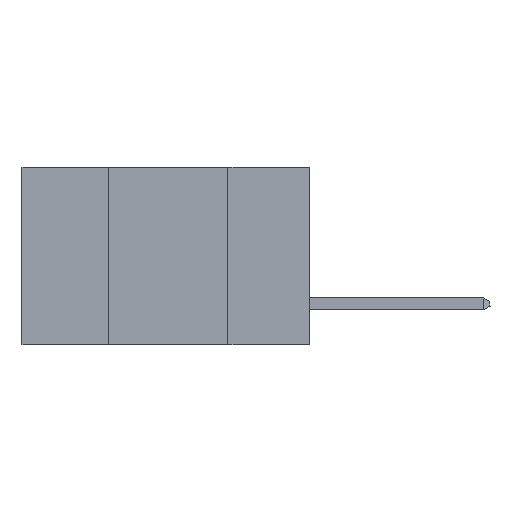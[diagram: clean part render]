
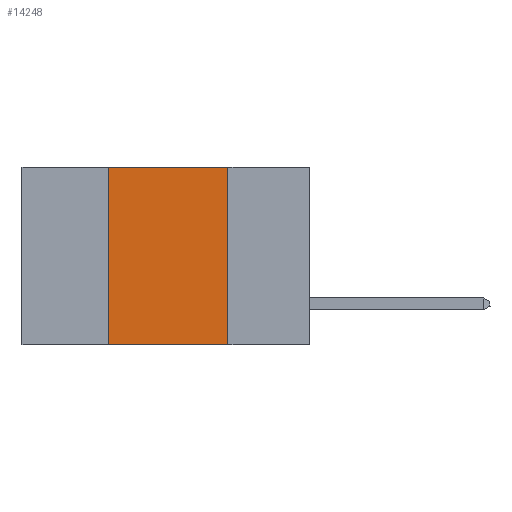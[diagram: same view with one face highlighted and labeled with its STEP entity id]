
A CAD part, left-side view. The second image highlights one B-rep face of the part: STEP entity #14248.
In plain terms, the highlighted planar face has unit normal (-1, 0, 0).
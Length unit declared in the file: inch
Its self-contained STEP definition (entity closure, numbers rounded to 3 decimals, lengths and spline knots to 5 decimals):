
#687 = AXIS2_PLACEMENT_3D ( 'NONE', #15454, #2867, #1609 ) ;
#1334 = EDGE_CURVE ( 'NONE', #13517, #1570, #4063, .T. ) ;
#1570 = VERTEX_POINT ( 'NONE', #13512 ) ;
#1609 = DIRECTION ( 'NONE',  ( 0., 0., -1. ) ) ;
#2159 = LINE ( 'NONE', #13536, #5321 ) ;
#2220 = CARTESIAN_POINT ( 'NONE',  ( 0., 0.42, -0.37 ) ) ;
#2588 = DIRECTION ( 'NONE',  ( 0., -1., 0. ) ) ;
#2867 = DIRECTION ( 'NONE',  ( 1., 0., 0. ) ) ;
#2921 = PLANE ( 'NONE',  #687 ) ;
#3475 = ORIENTED_EDGE ( 'NONE', *, *, #1334, .F. ) ;
#3502 = LINE ( 'NONE', #4851, #13552 ) ;
#4063 = LINE ( 'NONE', #8193, #14668 ) ;
#4851 = CARTESIAN_POINT ( 'NONE',  ( 0., 0.17, 0. ) ) ;
#5321 = VECTOR ( 'NONE', #14844, 39.37008 ) ;
#6093 = DIRECTION ( 'NONE',  ( 0., 0., -1. ) ) ;
#6824 = VERTEX_POINT ( 'NONE', #15093 ) ;
#7123 = CARTESIAN_POINT ( 'NONE',  ( 0., 0.17, 0. ) ) ;
#8193 = CARTESIAN_POINT ( 'NONE',  ( 0., 0.42, 0. ) ) ;
#8251 = DIRECTION ( 'NONE',  ( 0., 0., 1. ) ) ;
#8395 = VECTOR ( 'NONE', #2588, 39.37008 ) ;
#8502 = FACE_OUTER_BOUND ( 'NONE', #9067, .T. ) ;
#9067 = EDGE_LOOP ( 'NONE', ( #9069, #12252, #3475, #12492 ) ) ;
#9069 = ORIENTED_EDGE ( 'NONE', *, *, #9798, .F. ) ;
#9436 = EDGE_CURVE ( 'NONE', #1570, #12215, #2159, .T. ) ;
#9798 = EDGE_CURVE ( 'NONE', #12215, #6824, #3502, .T. ) ;
#11364 = EDGE_CURVE ( 'NONE', #13517, #6824, #15077, .T. ) ;
#12215 = VERTEX_POINT ( 'NONE', #7123 ) ;
#12252 = ORIENTED_EDGE ( 'NONE', *, *, #9436, .F. ) ;
#12492 = ORIENTED_EDGE ( 'NONE', *, *, #11364, .T. ) ;
#13512 = CARTESIAN_POINT ( 'NONE',  ( 0., 0.42, 0. ) ) ;
#13517 = VERTEX_POINT ( 'NONE', #2220 ) ;
#13536 = CARTESIAN_POINT ( 'NONE',  ( 0., 0.6, 0. ) ) ;
#13552 = VECTOR ( 'NONE', #6093, 39.37008 ) ;
#13936 = CARTESIAN_POINT ( 'NONE',  ( 0., 0.6, -0.37 ) ) ;
#14248 = ADVANCED_FACE ( 'NONE', ( #8502 ), #2921, .F. ) ;
#14668 = VECTOR ( 'NONE', #8251, 39.37008 ) ;
#14844 = DIRECTION ( 'NONE',  ( 0., -1., 0. ) ) ;
#15077 = LINE ( 'NONE', #13936, #8395 ) ;
#15093 = CARTESIAN_POINT ( 'NONE',  ( 0., 0.17, -0.37 ) ) ;
#15454 = CARTESIAN_POINT ( 'NONE',  ( 0., 0.6, 0. ) ) ;
